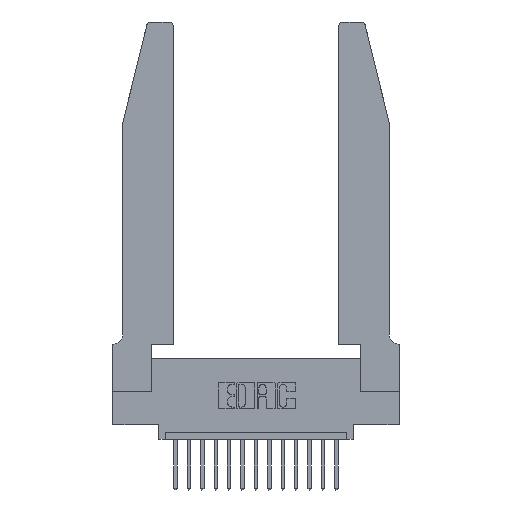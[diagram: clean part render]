
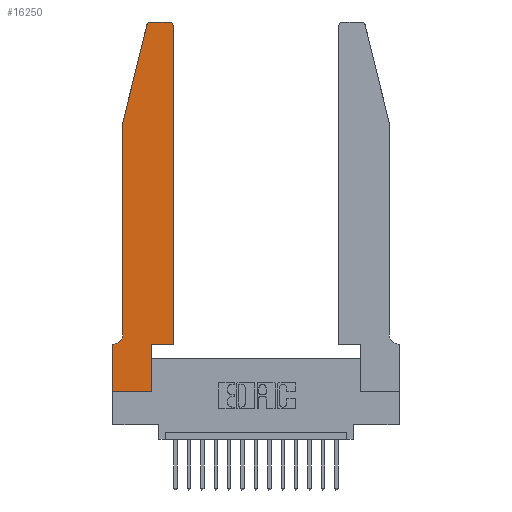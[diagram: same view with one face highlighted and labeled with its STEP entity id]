
A CAD part, top view. The second image highlights one B-rep face of the part: STEP entity #16250.
In plain terms, the highlighted planar face has unit normal (0, 0, 1).
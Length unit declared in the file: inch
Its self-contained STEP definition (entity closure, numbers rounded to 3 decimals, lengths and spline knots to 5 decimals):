
#422 = VERTEX_POINT ( 'NONE', #11464 ) ;
#426 = CARTESIAN_POINT ( 'NONE',  ( 0.4205, 2.72, 0.37 ) ) ;
#862 = ORIENTED_EDGE ( 'NONE', *, *, #15966, .T. ) ;
#872 = CARTESIAN_POINT ( 'NONE',  ( 0.0055, 0.35, 0.37 ) ) ;
#1513 = CIRCLE ( 'NONE', #4773, 0.07 ) ;
#1553 = DIRECTION ( 'NONE',  ( 0., 0., 1. ) ) ;
#1710 = VECTOR ( 'NONE', #12389, 39.37008 ) ;
#1819 = DIRECTION ( 'NONE',  ( 0., 0., 1. ) ) ;
#1864 = EDGE_CURVE ( 'NONE', #3726, #10374, #13712, .T. ) ;
#1918 = ORIENTED_EDGE ( 'NONE', *, *, #6516, .T. ) ;
#2377 = CARTESIAN_POINT ( 'NONE',  ( 0.284, 2.72, 0.37 ) ) ;
#3041 = ORIENTED_EDGE ( 'NONE', *, *, #9764, .T. ) ;
#3099 = EDGE_CURVE ( 'NONE', #17844, #16984, #17870, .T. ) ;
#3206 = ORIENTED_EDGE ( 'NONE', *, *, #10805, .T. ) ;
#3207 = LINE ( 'NONE', #12609, #7415 ) ;
#3337 = CARTESIAN_POINT ( 'NONE',  ( 0., 0., 0.37 ) ) ;
#3475 = DIRECTION ( 'NONE',  ( 0., 1., 0. ) ) ;
#3556 = EDGE_CURVE ( 'NONE', #5009, #7574, #11721, .T. ) ;
#3726 = VERTEX_POINT ( 'NONE', #8532 ) ;
#3785 = CARTESIAN_POINT ( 'NONE',  ( 0.0755, 2., 0.37 ) ) ;
#4043 = ORIENTED_EDGE ( 'NONE', *, *, #3099, .T. ) ;
#4262 = CARTESIAN_POINT ( 'NONE',  ( 0.4505, 0.35, 0.37 ) ) ;
#4437 = DIRECTION ( 'NONE',  ( 1., 0., 0. ) ) ;
#4734 = ORIENTED_EDGE ( 'NONE', *, *, #3556, .T. ) ;
#4773 = AXIS2_PLACEMENT_3D ( 'NONE', #5517, #15662, #15534 ) ;
#5009 = VERTEX_POINT ( 'NONE', #5508 ) ;
#5088 = ORIENTED_EDGE ( 'NONE', *, *, #1864, .T. ) ;
#5240 = DIRECTION ( 'NONE',  ( 0., 0., 1. ) ) ;
#5354 = DIRECTION ( 'NONE',  ( -0.239, -0.971, 0. ) ) ;
#5483 = VERTEX_POINT ( 'NONE', #6196 ) ;
#5508 = CARTESIAN_POINT ( 'NONE',  ( 0.284, 2.75, 0.37 ) ) ;
#5517 = CARTESIAN_POINT ( 'NONE',  ( 0.0055, 0.42, 0.37 ) ) ;
#5719 = LINE ( 'NONE', #3785, #14907 ) ;
#5908 = ORIENTED_EDGE ( 'NONE', *, *, #13930, .T. ) ;
#6196 = CARTESIAN_POINT ( 'NONE',  ( 0.4205, 2.75, 0.37 ) ) ;
#6516 = EDGE_CURVE ( 'NONE', #5483, #5009, #15493, .T. ) ;
#6631 = ORIENTED_EDGE ( 'NONE', *, *, #12386, .T. ) ;
#6706 = CARTESIAN_POINT ( 'NONE',  ( 0.2865, 0.35, 0.37 ) ) ;
#7363 = VECTOR ( 'NONE', #17440, 39.37008 ) ;
#7415 = VECTOR ( 'NONE', #10972, 39.37008 ) ;
#7441 = ORIENTED_EDGE ( 'NONE', *, *, #17893, .T. ) ;
#7574 = VERTEX_POINT ( 'NONE', #16564 ) ;
#8261 = CIRCLE ( 'NONE', #17241, 0.03 ) ;
#8532 = CARTESIAN_POINT ( 'NONE',  ( 0., 0.35, 0.37 ) ) ;
#8687 = CARTESIAN_POINT ( 'NONE',  ( 0., 0., 0.37 ) ) ;
#8731 = VECTOR ( 'NONE', #9892, 39.37008 ) ;
#8872 = CARTESIAN_POINT ( 'NONE',  ( 0.0755, 2., 0.37 ) ) ;
#8898 = AXIS2_PLACEMENT_3D ( 'NONE', #2377, #5240, #16832 ) ;
#8968 = PLANE ( 'NONE',  #12024 ) ;
#9077 = EDGE_LOOP ( 'NONE', ( #1918, #4734, #6631, #17811, #7441, #3206, #5088, #5908, #4043, #862, #3041, #17931 ) ) ;
#9482 = CARTESIAN_POINT ( 'NONE',  ( 0.2865, 0., 0.37 ) ) ;
#9695 = VERTEX_POINT ( 'NONE', #4262 ) ;
#9764 = EDGE_CURVE ( 'NONE', #9695, #13288, #18365, .T. ) ;
#9892 = DIRECTION ( 'NONE',  ( -1., 0., 0. ) ) ;
#10021 = VECTOR ( 'NONE', #3475, 39.37008 ) ;
#10344 = CARTESIAN_POINT ( 'NONE',  ( 0., 0.35, 0.37 ) ) ;
#10374 = VERTEX_POINT ( 'NONE', #8687 ) ;
#10805 = EDGE_CURVE ( 'NONE', #18173, #3726, #16960, .T. ) ;
#10834 = CARTESIAN_POINT ( 'NONE',  ( 0.4505, 2.72, 0.37 ) ) ;
#10972 = DIRECTION ( 'NONE',  ( 1., 0., 0. ) ) ;
#11128 = CARTESIAN_POINT ( 'NONE',  ( 0.2605, 2.75, 0.37 ) ) ;
#11464 = CARTESIAN_POINT ( 'NONE',  ( 0.0755, 0.42, 0.37 ) ) ;
#11533 = DIRECTION ( 'NONE',  ( 1., 0., 0. ) ) ;
#11721 = CIRCLE ( 'NONE', #8898, 0.03 ) ;
#12024 = AXIS2_PLACEMENT_3D ( 'NONE', #10344, #1553, #11533 ) ;
#12386 = EDGE_CURVE ( 'NONE', #7574, #17389, #5719, .T. ) ;
#12389 = DIRECTION ( 'NONE',  ( 0., 1., 0. ) ) ;
#12609 = CARTESIAN_POINT ( 'NONE',  ( 0.4505, 0.35, 0.37 ) ) ;
#12633 = CARTESIAN_POINT ( 'NONE',  ( 0., 0., 0.37 ) ) ;
#12638 = CARTESIAN_POINT ( 'NONE',  ( 0.2865, 0.35, 0.37 ) ) ;
#12819 = CARTESIAN_POINT ( 'NONE',  ( 0.0755, 2., 0.37 ) ) ;
#13104 = VECTOR ( 'NONE', #15971, 39.37008 ) ;
#13288 = VERTEX_POINT ( 'NONE', #10834 ) ;
#13348 = CARTESIAN_POINT ( 'NONE',  ( 0.4505, 0.35, 0.37 ) ) ;
#13712 = LINE ( 'NONE', #12633, #17117 ) ;
#13930 = EDGE_CURVE ( 'NONE', #10374, #17844, #18007, .T. ) ;
#14117 = FACE_OUTER_BOUND ( 'NONE', #9077, .T. ) ;
#14907 = VECTOR ( 'NONE', #5354, 39.37008 ) ;
#15467 = EDGE_CURVE ( 'NONE', #17389, #422, #17499, .T. ) ;
#15493 = LINE ( 'NONE', #11128, #8731 ) ;
#15534 = DIRECTION ( 'NONE',  ( -1., 0., 0. ) ) ;
#15662 = DIRECTION ( 'NONE',  ( 0., 0., -1. ) ) ;
#15966 = EDGE_CURVE ( 'NONE', #16984, #9695, #3207, .T. ) ;
#15971 = DIRECTION ( 'NONE',  ( -1., 0., 0. ) ) ;
#16128 = DIRECTION ( 'NONE',  ( 1., 0., 0. ) ) ;
#16199 = EDGE_CURVE ( 'NONE', #13288, #5483, #8261, .T. ) ;
#16250 = ADVANCED_FACE ( 'NONE', ( #14117 ), #8968, .T. ) ;
#16564 = CARTESIAN_POINT ( 'NONE',  ( 0.25487, 2.72718, 0.37 ) ) ;
#16832 = DIRECTION ( 'NONE',  ( 1., 0., 0. ) ) ;
#16960 = LINE ( 'NONE', #17492, #13104 ) ;
#16984 = VERTEX_POINT ( 'NONE', #6706 ) ;
#17009 = DIRECTION ( 'NONE',  ( 0., -1., 0. ) ) ;
#17117 = VECTOR ( 'NONE', #17009, 39.37008 ) ;
#17241 = AXIS2_PLACEMENT_3D ( 'NONE', #426, #1819, #4437 ) ;
#17321 = VECTOR ( 'NONE', #16128, 39.37008 ) ;
#17389 = VERTEX_POINT ( 'NONE', #12819 ) ;
#17440 = DIRECTION ( 'NONE',  ( 0., -1., 0. ) ) ;
#17492 = CARTESIAN_POINT ( 'NONE',  ( 0.0755, 0.35, 0.37 ) ) ;
#17499 = LINE ( 'NONE', #8872, #7363 ) ;
#17811 = ORIENTED_EDGE ( 'NONE', *, *, #15467, .T. ) ;
#17844 = VERTEX_POINT ( 'NONE', #9482 ) ;
#17870 = LINE ( 'NONE', #12638, #1710 ) ;
#17893 = EDGE_CURVE ( 'NONE', #422, #18173, #1513, .T. ) ;
#17931 = ORIENTED_EDGE ( 'NONE', *, *, #16199, .T. ) ;
#18007 = LINE ( 'NONE', #3337, #17321 ) ;
#18173 = VERTEX_POINT ( 'NONE', #872 ) ;
#18365 = LINE ( 'NONE', #13348, #10021 ) ;
